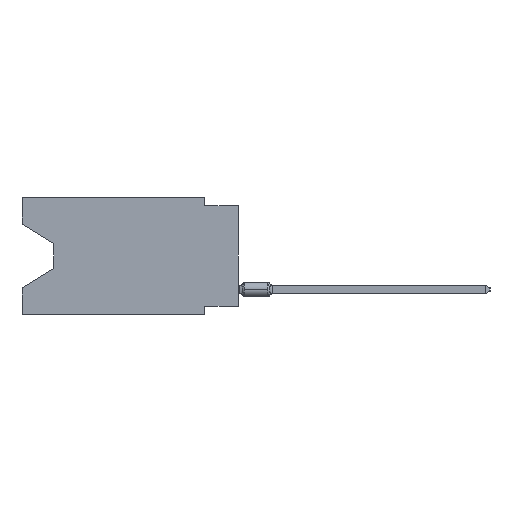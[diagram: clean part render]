
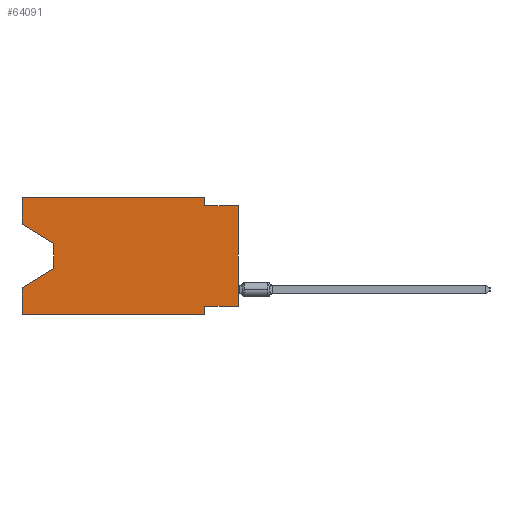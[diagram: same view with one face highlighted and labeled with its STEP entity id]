
A CAD part, left-side view. The second image highlights one B-rep face of the part: STEP entity #64091.
In plain terms, the highlighted planar face has unit normal (-1, 0, 0).
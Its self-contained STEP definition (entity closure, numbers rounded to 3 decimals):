
#405 = EDGE_CURVE ( 'NONE', #59306, #34402, #98587, .T. ) ;
#544 = LINE ( 'NONE', #98916, #52129 ) ;
#755 = VERTEX_POINT ( 'NONE', #78742 ) ;
#838 = ORIENTED_EDGE ( 'NONE', *, *, #66851, .F. ) ;
#1069 = DIRECTION ( 'NONE',  ( 0., 0., 1. ) ) ;
#2146 = CARTESIAN_POINT ( 'NONE',  ( 0., 0., -8.255 ) ) ;
#2560 = EDGE_CURVE ( 'NONE', #89558, #9040, #83836, .T. ) ;
#2806 = EDGE_CURVE ( 'NONE', #50348, #51148, #87526, .T. ) ;
#4139 = DIRECTION ( 'NONE',  ( 0., -0.855, -0.519 ) ) ;
#6090 = DIRECTION ( 'NONE',  ( 0., 0., 1. ) ) ;
#7524 = CARTESIAN_POINT ( 'NONE',  ( 0., 2.54, 0. ) ) ;
#7780 = FACE_OUTER_BOUND ( 'NONE', #31656, .T. ) ;
#9040 = VERTEX_POINT ( 'NONE', #95696 ) ;
#9599 = CARTESIAN_POINT ( 'NONE',  ( 0., 0., 0. ) ) ;
#9623 = LINE ( 'NONE', #34235, #76030 ) ;
#10563 = CARTESIAN_POINT ( 'NONE',  ( 0., 16.383, -8.89 ) ) ;
#11351 = ORIENTED_EDGE ( 'NONE', *, *, #2560, .T. ) ;
#14780 = CARTESIAN_POINT ( 'NONE',  ( 0., 16.383, -2.038 ) ) ;
#15138 = LINE ( 'NONE', #30681, #70020 ) ;
#15510 = VECTOR ( 'NONE', #104336, 1000. ) ;
#15979 = ORIENTED_EDGE ( 'NONE', *, *, #2806, .T. ) ;
#16324 = DIRECTION ( 'NONE',  ( 0., 0., -1. ) ) ;
#18841 = CARTESIAN_POINT ( 'NONE',  ( 0., 16.383, -8.89 ) ) ;
#19072 = ORIENTED_EDGE ( 'NONE', *, *, #405, .F. ) ;
#23771 = VERTEX_POINT ( 'NONE', #68175 ) ;
#24339 = EDGE_CURVE ( 'NONE', #72815, #102140, #30572, .T. ) ;
#25340 = DIRECTION ( 'NONE',  ( 0., -1., 0. ) ) ;
#25939 = DIRECTION ( 'NONE',  ( 1., 0., 0. ) ) ;
#30080 = VECTOR ( 'NONE', #43858, 1000. ) ;
#30572 = LINE ( 'NONE', #48738, #15510 ) ;
#30681 = CARTESIAN_POINT ( 'NONE',  ( 0., 16.383, 0. ) ) ;
#31609 = LINE ( 'NONE', #7524, #91404 ) ;
#31656 = EDGE_LOOP ( 'NONE', ( #15979, #105268, #50087, #98083, #11351, #838, #79823, #43075, #19072, #77319, #37494, #81749 ) ) ;
#31746 = LINE ( 'NONE', #73412, #78219 ) ;
#34235 = CARTESIAN_POINT ( 'NONE',  ( 0., 16.383, 0. ) ) ;
#34402 = VERTEX_POINT ( 'NONE', #39266 ) ;
#37494 = ORIENTED_EDGE ( 'NONE', *, *, #24339, .F. ) ;
#37862 = EDGE_CURVE ( 'NONE', #53006, #34402, #58818, .T. ) ;
#38982 = EDGE_CURVE ( 'NONE', #102140, #59306, #31609, .T. ) ;
#39266 = CARTESIAN_POINT ( 'NONE',  ( 0., 0., -0.635 ) ) ;
#40162 = DIRECTION ( 'NONE',  ( 0., 0., -1. ) ) ;
#41005 = LINE ( 'NONE', #54971, #46565 ) ;
#43075 = ORIENTED_EDGE ( 'NONE', *, *, #37862, .T. ) ;
#43858 = DIRECTION ( 'NONE',  ( 0., 0.855, -0.519 ) ) ;
#46350 = CARTESIAN_POINT ( 'NONE',  ( 0., 16.383, 0. ) ) ;
#46565 = VECTOR ( 'NONE', #79530, 1000. ) ;
#47803 = DIRECTION ( 'NONE',  ( 0., 1., 0. ) ) ;
#48669 = EDGE_CURVE ( 'NONE', #51148, #23771, #544, .T. ) ;
#48738 = CARTESIAN_POINT ( 'NONE',  ( 0., 16.383, 0. ) ) ;
#50087 = ORIENTED_EDGE ( 'NONE', *, *, #82728, .T. ) ;
#50348 = VERTEX_POINT ( 'NONE', #102580 ) ;
#51148 = VERTEX_POINT ( 'NONE', #103380 ) ;
#52129 = VECTOR ( 'NONE', #66841, 1000. ) ;
#52824 = DIRECTION ( 'NONE',  ( 0., -1., 0. ) ) ;
#53006 = VERTEX_POINT ( 'NONE', #2146 ) ;
#54971 = CARTESIAN_POINT ( 'NONE',  ( 0., 2.54, -8.89 ) ) ;
#56638 = CARTESIAN_POINT ( 'NONE',  ( 0., 2.54, 0. ) ) ;
#58818 = LINE ( 'NONE', #9599, #58976 ) ;
#58840 = DIRECTION ( 'NONE',  ( 0., 0., 1. ) ) ;
#58976 = VECTOR ( 'NONE', #1069, 1000. ) ;
#59306 = VERTEX_POINT ( 'NONE', #74676 ) ;
#59574 = VECTOR ( 'NONE', #52824, 1000. ) ;
#63215 = EDGE_CURVE ( 'NONE', #89558, #755, #15138, .T. ) ;
#64091 = ADVANCED_FACE ( 'NONE', ( #7780 ), #86979, .F. ) ;
#66345 = LINE ( 'NONE', #98950, #30080 ) ;
#66841 = DIRECTION ( 'NONE',  ( 0., 0., -1. ) ) ;
#66851 = EDGE_CURVE ( 'NONE', #79807, #9040, #41005, .T. ) ;
#67989 = CARTESIAN_POINT ( 'NONE',  ( 0., 2.54, -8.255 ) ) ;
#68175 = CARTESIAN_POINT ( 'NONE',  ( 0., 13.97, -5.385 ) ) ;
#70020 = VECTOR ( 'NONE', #6090, 1000. ) ;
#72815 = VERTEX_POINT ( 'NONE', #95355 ) ;
#73412 = CARTESIAN_POINT ( 'NONE',  ( 0., 0., -8.255 ) ) ;
#74676 = CARTESIAN_POINT ( 'NONE',  ( 0., 2.54, -0.635 ) ) ;
#76030 = VECTOR ( 'NONE', #58840, 1000. ) ;
#77319 = ORIENTED_EDGE ( 'NONE', *, *, #38982, .F. ) ;
#78219 = VECTOR ( 'NONE', #47803, 1000. ) ;
#78742 = CARTESIAN_POINT ( 'NONE',  ( 0., 16.383, -6.852 ) ) ;
#79530 = DIRECTION ( 'NONE',  ( 0., 0., -1. ) ) ;
#79807 = VERTEX_POINT ( 'NONE', #67989 ) ;
#79823 = ORIENTED_EDGE ( 'NONE', *, *, #101282, .F. ) ;
#81718 = EDGE_CURVE ( 'NONE', #50348, #72815, #9623, .T. ) ;
#81749 = ORIENTED_EDGE ( 'NONE', *, *, #81718, .F. ) ;
#82728 = EDGE_CURVE ( 'NONE', #23771, #755, #66345, .T. ) ;
#83836 = LINE ( 'NONE', #10563, #59574 ) ;
#86979 = PLANE ( 'NONE',  #95739 ) ;
#87526 = LINE ( 'NONE', #14780, #97198 ) ;
#88496 = CARTESIAN_POINT ( 'NONE',  ( 0., 0., -0.635 ) ) ;
#89558 = VERTEX_POINT ( 'NONE', #18841 ) ;
#91404 = VECTOR ( 'NONE', #40162, 1000. ) ;
#95355 = CARTESIAN_POINT ( 'NONE',  ( 0., 16.383, 0. ) ) ;
#95696 = CARTESIAN_POINT ( 'NONE',  ( 0., 2.54, -8.89 ) ) ;
#95739 = AXIS2_PLACEMENT_3D ( 'NONE', #46350, #25939, #16324 ) ;
#96794 = VECTOR ( 'NONE', #25340, 1000. ) ;
#97198 = VECTOR ( 'NONE', #4139, 1000. ) ;
#98083 = ORIENTED_EDGE ( 'NONE', *, *, #63215, .F. ) ;
#98587 = LINE ( 'NONE', #88496, #96794 ) ;
#98916 = CARTESIAN_POINT ( 'NONE',  ( 0., 13.97, -3.505 ) ) ;
#98950 = CARTESIAN_POINT ( 'NONE',  ( 0., 13.97, -5.385 ) ) ;
#101282 = EDGE_CURVE ( 'NONE', #53006, #79807, #31746, .T. ) ;
#102140 = VERTEX_POINT ( 'NONE', #56638 ) ;
#102580 = CARTESIAN_POINT ( 'NONE',  ( 0., 16.383, -2.038 ) ) ;
#103380 = CARTESIAN_POINT ( 'NONE',  ( 0., 13.97, -3.505 ) ) ;
#104336 = DIRECTION ( 'NONE',  ( 0., -1., 0. ) ) ;
#105268 = ORIENTED_EDGE ( 'NONE', *, *, #48669, .T. ) ;
